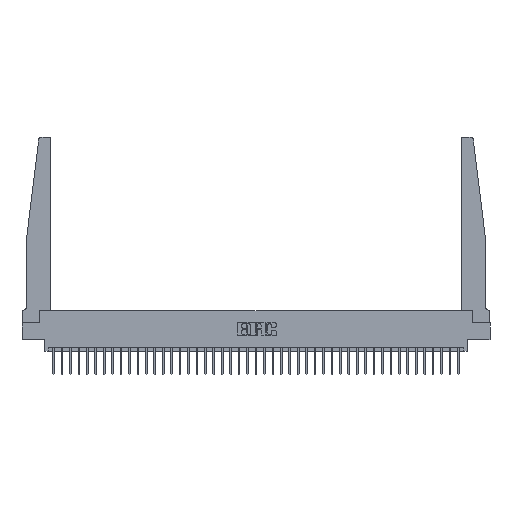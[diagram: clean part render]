
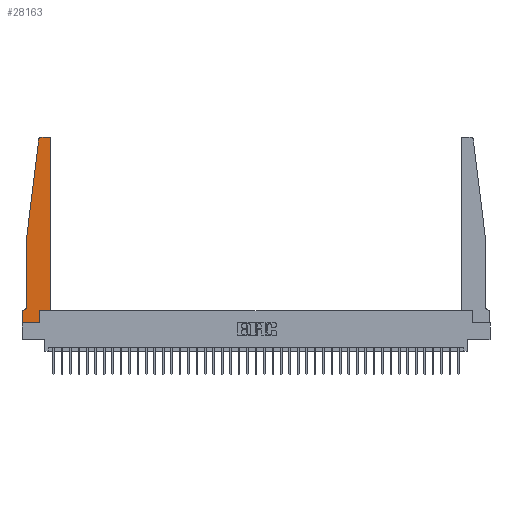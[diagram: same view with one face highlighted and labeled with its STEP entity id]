
A CAD part, top view. The second image highlights one B-rep face of the part: STEP entity #28163.
In plain terms, the highlighted planar face has unit normal (0, 0, 1).
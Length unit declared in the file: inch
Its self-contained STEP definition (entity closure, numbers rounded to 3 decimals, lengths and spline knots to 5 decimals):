
#191 = CIRCLE ( 'NONE', #21410, 0.03 ) ;
#243 = EDGE_CURVE ( 'NONE', #1889, #20433, #32525, .T. ) ;
#349 = DIRECTION ( 'NONE',  ( 0., 0., 1. ) ) ;
#939 = CARTESIAN_POINT ( 'NONE',  ( 0., 0., 0.37 ) ) ;
#1001 = CARTESIAN_POINT ( 'NONE',  ( 0.27653, 2.72, 0.37 ) ) ;
#1238 = VERTEX_POINT ( 'NONE', #5657 ) ;
#1305 = CARTESIAN_POINT ( 'NONE',  ( 0., 0.1875, 0.37 ) ) ;
#1690 = EDGE_CURVE ( 'NONE', #16274, #33813, #27198, .T. ) ;
#1889 = VERTEX_POINT ( 'NONE', #12410 ) ;
#1942 = CARTESIAN_POINT ( 'NONE',  ( 0., 0., 0.37 ) ) ;
#2700 = VECTOR ( 'NONE', #30220, 39.37008 ) ;
#3271 = EDGE_CURVE ( 'NONE', #31766, #25860, #16018, .T. ) ;
#3861 = ORIENTED_EDGE ( 'NONE', *, *, #10407, .T. ) ;
#4229 = CARTESIAN_POINT ( 'NONE',  ( 0.395, 2.75, 0.37 ) ) ;
#4589 = ORIENTED_EDGE ( 'NONE', *, *, #12545, .T. ) ;
#4895 = ORIENTED_EDGE ( 'NONE', *, *, #243, .T. ) ;
#5017 = CARTESIAN_POINT ( 'NONE',  ( 0.065, 1.25, 0.37 ) ) ;
#5150 = VECTOR ( 'NONE', #14740, 39.37008 ) ;
#5657 = CARTESIAN_POINT ( 'NONE',  ( 0.065, 1.25, 0.37 ) ) ;
#6428 = LINE ( 'NONE', #17321, #20707 ) ;
#6714 = DIRECTION ( 'NONE',  ( 1., 0., 0. ) ) ;
#7406 = CARTESIAN_POINT ( 'NONE',  ( 0.2605, 0., 0.37 ) ) ;
#8807 = DIRECTION ( 'NONE',  ( 1., 0., 0. ) ) ;
#9317 = CARTESIAN_POINT ( 'NONE',  ( 0.065, 0.2375, 0.37 ) ) ;
#9519 = AXIS2_PLACEMENT_3D ( 'NONE', #32782, #18215, #23932 ) ;
#9631 = CARTESIAN_POINT ( 'NONE',  ( 0.2605, 0.18, 0.37 ) ) ;
#9640 = EDGE_CURVE ( 'NONE', #1238, #29879, #23831, .T. ) ;
#10029 = ORIENTED_EDGE ( 'NONE', *, *, #1690, .T. ) ;
#10256 = VERTEX_POINT ( 'NONE', #15067 ) ;
#10397 = DIRECTION ( 'NONE',  ( -1., 0., 0. ) ) ;
#10407 = EDGE_CURVE ( 'NONE', #20433, #16274, #18072, .T. ) ;
#10952 = VECTOR ( 'NONE', #24819, 39.37008 ) ;
#11874 = EDGE_CURVE ( 'NONE', #33813, #13312, #18975, .T. ) ;
#12243 = DIRECTION ( 'NONE',  ( 0., 0., 1. ) ) ;
#12330 = ORIENTED_EDGE ( 'NONE', *, *, #11874, .T. ) ;
#12410 = CARTESIAN_POINT ( 'NONE',  ( 0.015, 0.1875, 0.37 ) ) ;
#12439 = EDGE_CURVE ( 'NONE', #25167, #31766, #13773, .T. ) ;
#12545 = EDGE_CURVE ( 'NONE', #29879, #1889, #23879, .T. ) ;
#12805 = LINE ( 'NONE', #24752, #23262 ) ;
#13188 = DIRECTION ( 'NONE',  ( 1., 0., 0. ) ) ;
#13312 = VERTEX_POINT ( 'NONE', #9631 ) ;
#13773 = LINE ( 'NONE', #33333, #10952 ) ;
#14280 = CARTESIAN_POINT ( 'NONE',  ( 0.425, 2.72, 0.37 ) ) ;
#14500 = DIRECTION ( 'NONE',  ( -1., 0., 0. ) ) ;
#14740 = DIRECTION ( 'NONE',  ( 0., -1., 0. ) ) ;
#15067 = CARTESIAN_POINT ( 'NONE',  ( 0.24675, 2.72367, 0.37 ) ) ;
#16018 = CIRCLE ( 'NONE', #9519, 0.03 ) ;
#16089 = DIRECTION ( 'NONE',  ( 0., -1., 0. ) ) ;
#16274 = VERTEX_POINT ( 'NONE', #27145 ) ;
#17321 = CARTESIAN_POINT ( 'NONE',  ( 0.425, 0.18, 0.37 ) ) ;
#17463 = VECTOR ( 'NONE', #16089, 39.37008 ) ;
#17613 = DIRECTION ( 'NONE',  ( -1., 0., 0. ) ) ;
#18072 = LINE ( 'NONE', #939, #5150 ) ;
#18215 = DIRECTION ( 'NONE',  ( 0., 0., 1. ) ) ;
#18975 = LINE ( 'NONE', #19167, #2700 ) ;
#19167 = CARTESIAN_POINT ( 'NONE',  ( 0.2605, 0.18, 0.37 ) ) ;
#19530 = ORIENTED_EDGE ( 'NONE', *, *, #12439, .T. ) ;
#19986 = EDGE_CURVE ( 'NONE', #20995, #10256, #191, .T. ) ;
#20142 = CARTESIAN_POINT ( 'NONE',  ( 0.425, 0.18, 0.37 ) ) ;
#20433 = VERTEX_POINT ( 'NONE', #1305 ) ;
#20707 = VECTOR ( 'NONE', #28367, 39.37008 ) ;
#20738 = CARTESIAN_POINT ( 'NONE',  ( 0.015, 0.2375, 0.37 ) ) ;
#20913 = LINE ( 'NONE', #32170, #25031 ) ;
#20995 = VERTEX_POINT ( 'NONE', #27259 ) ;
#21347 = ORIENTED_EDGE ( 'NONE', *, *, #33456, .T. ) ;
#21410 = AXIS2_PLACEMENT_3D ( 'NONE', #1001, #12243, #6714 ) ;
#21633 = ORIENTED_EDGE ( 'NONE', *, *, #19986, .T. ) ;
#22427 = VECTOR ( 'NONE', #10397, 39.37008 ) ;
#23262 = VECTOR ( 'NONE', #26822, 39.37008 ) ;
#23831 = LINE ( 'NONE', #5017, #17463 ) ;
#23879 = CIRCLE ( 'NONE', #28598, 0.05 ) ;
#23932 = DIRECTION ( 'NONE',  ( 1., 0., 0. ) ) ;
#24752 = CARTESIAN_POINT ( 'NONE',  ( 0.065, 1.25, 0.37 ) ) ;
#24819 = DIRECTION ( 'NONE',  ( 0., 1., 0. ) ) ;
#25031 = VECTOR ( 'NONE', #17613, 39.37008 ) ;
#25167 = VERTEX_POINT ( 'NONE', #20142 ) ;
#25601 = PLANE ( 'NONE',  #34847 ) ;
#25676 = ORIENTED_EDGE ( 'NONE', *, *, #3271, .T. ) ;
#25860 = VERTEX_POINT ( 'NONE', #4229 ) ;
#26297 = DIRECTION ( 'NONE',  ( 0., 0., -1. ) ) ;
#26822 = DIRECTION ( 'NONE',  ( -0.122, -0.992, 0. ) ) ;
#27145 = CARTESIAN_POINT ( 'NONE',  ( 0., 0., 0.37 ) ) ;
#27198 = LINE ( 'NONE', #1942, #28854 ) ;
#27259 = CARTESIAN_POINT ( 'NONE',  ( 0.27653, 2.75, 0.37 ) ) ;
#28133 = EDGE_CURVE ( 'NONE', #13312, #25167, #6428, .T. ) ;
#28163 = ADVANCED_FACE ( 'NONE', ( #28739 ), #25601, .T. ) ;
#28367 = DIRECTION ( 'NONE',  ( 1., 0., 0. ) ) ;
#28598 = AXIS2_PLACEMENT_3D ( 'NONE', #20738, #26297, #14500 ) ;
#28739 = FACE_OUTER_BOUND ( 'NONE', #30256, .T. ) ;
#28854 = VECTOR ( 'NONE', #13188, 39.37008 ) ;
#29100 = CARTESIAN_POINT ( 'NONE',  ( 0., 0.1875, 0.37 ) ) ;
#29879 = VERTEX_POINT ( 'NONE', #9317 ) ;
#30220 = DIRECTION ( 'NONE',  ( 0., 1., 0. ) ) ;
#30256 = EDGE_LOOP ( 'NONE', ( #33347, #21633, #21347, #35905, #4589, #4895, #3861, #10029, #12330, #33331, #19530, #25676 ) ) ;
#31766 = VERTEX_POINT ( 'NONE', #14280 ) ;
#31981 = EDGE_CURVE ( 'NONE', #25860, #20995, #20913, .T. ) ;
#32170 = CARTESIAN_POINT ( 'NONE',  ( 0.25, 2.75, 0.37 ) ) ;
#32525 = LINE ( 'NONE', #35656, #22427 ) ;
#32782 = CARTESIAN_POINT ( 'NONE',  ( 0.395, 2.72, 0.37 ) ) ;
#33331 = ORIENTED_EDGE ( 'NONE', *, *, #28133, .T. ) ;
#33333 = CARTESIAN_POINT ( 'NONE',  ( 0.425, 0.18, 0.37 ) ) ;
#33347 = ORIENTED_EDGE ( 'NONE', *, *, #31981, .T. ) ;
#33456 = EDGE_CURVE ( 'NONE', #10256, #1238, #12805, .T. ) ;
#33813 = VERTEX_POINT ( 'NONE', #7406 ) ;
#34847 = AXIS2_PLACEMENT_3D ( 'NONE', #29100, #349, #8807 ) ;
#35656 = CARTESIAN_POINT ( 'NONE',  ( 0.065, 0.1875, 0.37 ) ) ;
#35905 = ORIENTED_EDGE ( 'NONE', *, *, #9640, .T. ) ;
